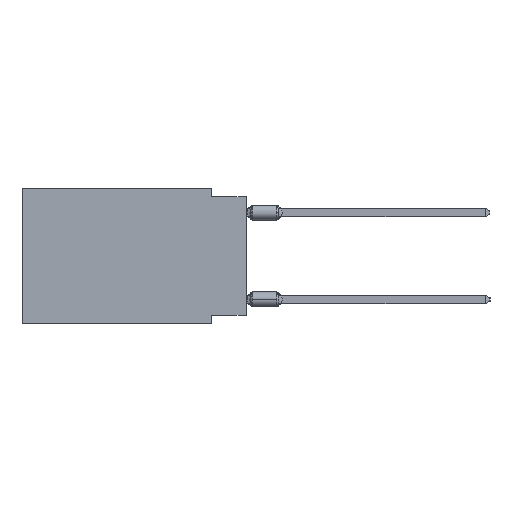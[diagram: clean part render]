
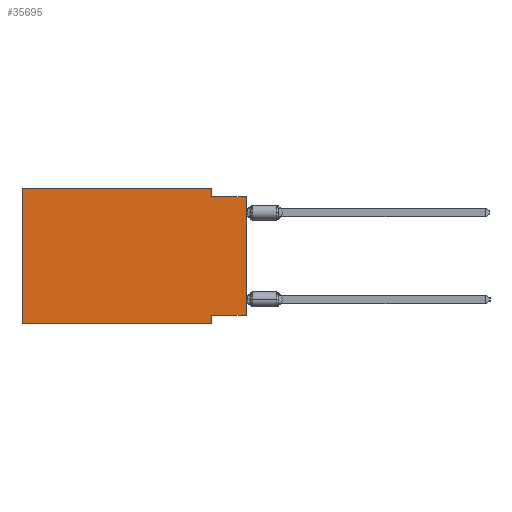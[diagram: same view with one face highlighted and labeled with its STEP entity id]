
A CAD part, left-side view. The second image highlights one B-rep face of the part: STEP entity #35695.
In plain terms, the highlighted planar face has unit normal (-1, 0, 0).
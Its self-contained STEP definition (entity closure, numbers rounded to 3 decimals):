
#551 = EDGE_CURVE ( 'NONE', #41948, #16310, #34120, .T. ) ;
#929 = DIRECTION ( 'NONE',  ( 0., 0., 1. ) ) ;
#3057 = ORIENTED_EDGE ( 'NONE', *, *, #26058, .F. ) ;
#3910 = CARTESIAN_POINT ( 'NONE',  ( 0., 2.54, -9.906 ) ) ;
#4034 = LINE ( 'NONE', #36126, #18903 ) ;
#4175 = VECTOR ( 'NONE', #14266, 1000. ) ;
#4250 = VERTEX_POINT ( 'NONE', #23758 ) ;
#4418 = DIRECTION ( 'NONE',  ( 0., -1., 0. ) ) ;
#5272 = ORIENTED_EDGE ( 'NONE', *, *, #21937, .F. ) ;
#5282 = CARTESIAN_POINT ( 'NONE',  ( 0., 2.54, 0. ) ) ;
#10532 = VECTOR ( 'NONE', #23453, 1000. ) ;
#10902 = PLANE ( 'NONE',  #42151 ) ;
#11302 = VECTOR ( 'NONE', #32524, 1000. ) ;
#14081 = VERTEX_POINT ( 'NONE', #3910 ) ;
#14266 = DIRECTION ( 'NONE',  ( 0., 1., 0. ) ) ;
#15259 = FACE_OUTER_BOUND ( 'NONE', #35864, .T. ) ;
#15515 = LINE ( 'NONE', #34306, #42172 ) ;
#15875 = VERTEX_POINT ( 'NONE', #19026 ) ;
#16050 = CARTESIAN_POINT ( 'NONE',  ( 0., 16.383, 0. ) ) ;
#16310 = VERTEX_POINT ( 'NONE', #20980 ) ;
#16678 = CARTESIAN_POINT ( 'NONE',  ( 0., 2.54, 0. ) ) ;
#16732 = LINE ( 'NONE', #36008, #33087 ) ;
#17043 = VECTOR ( 'NONE', #48157, 1000. ) ;
#18903 = VECTOR ( 'NONE', #929, 1000. ) ;
#19026 = CARTESIAN_POINT ( 'NONE',  ( 0., 0., -9.271 ) ) ;
#20980 = CARTESIAN_POINT ( 'NONE',  ( 0., 0., -0.635 ) ) ;
#21937 = EDGE_CURVE ( 'NONE', #40856, #30535, #4034, .T. ) ;
#22571 = CARTESIAN_POINT ( 'NONE',  ( 0., 0., -0.635 ) ) ;
#22885 = VECTOR ( 'NONE', #46199, 1000. ) ;
#23201 = LINE ( 'NONE', #26546, #10532 ) ;
#23453 = DIRECTION ( 'NONE',  ( 0., 0., 1. ) ) ;
#23758 = CARTESIAN_POINT ( 'NONE',  ( 0., 2.54, -9.271 ) ) ;
#24094 = CARTESIAN_POINT ( 'NONE',  ( 0., 16.383, 0. ) ) ;
#25014 = LINE ( 'NONE', #16050, #17043 ) ;
#26013 = ORIENTED_EDGE ( 'NONE', *, *, #44703, .F. ) ;
#26058 = EDGE_CURVE ( 'NONE', #4250, #14081, #15515, .T. ) ;
#26546 = CARTESIAN_POINT ( 'NONE',  ( 0., 0., 0. ) ) ;
#26577 = CARTESIAN_POINT ( 'NONE',  ( 0., 16.383, 0. ) ) ;
#28498 = ORIENTED_EDGE ( 'NONE', *, *, #551, .F. ) ;
#30317 = VERTEX_POINT ( 'NONE', #16678 ) ;
#30535 = VERTEX_POINT ( 'NONE', #24094 ) ;
#30918 = DIRECTION ( 'NONE',  ( 0., 0., -1. ) ) ;
#32524 = DIRECTION ( 'NONE',  ( 0., 0., -1. ) ) ;
#33087 = VECTOR ( 'NONE', #4418, 1000. ) ;
#34120 = LINE ( 'NONE', #22571, #22885 ) ;
#34306 = CARTESIAN_POINT ( 'NONE',  ( 0., 2.54, -9.906 ) ) ;
#34612 = ORIENTED_EDGE ( 'NONE', *, *, #45403, .T. ) ;
#34813 = DIRECTION ( 'NONE',  ( 0., 0., -1. ) ) ;
#35695 = ADVANCED_FACE ( 'NONE', ( #15259 ), #10902, .F. ) ;
#35864 = EDGE_LOOP ( 'NONE', ( #34612, #28498, #26013, #45335, #5272, #40911, #3057, #37621 ) ) ;
#36008 = CARTESIAN_POINT ( 'NONE',  ( 0., 16.383, -9.906 ) ) ;
#36126 = CARTESIAN_POINT ( 'NONE',  ( 0., 16.383, 0. ) ) ;
#37117 = EDGE_CURVE ( 'NONE', #40856, #14081, #16732, .T. ) ;
#37621 = ORIENTED_EDGE ( 'NONE', *, *, #50112, .F. ) ;
#37654 = LINE ( 'NONE', #45623, #4175 ) ;
#38395 = CARTESIAN_POINT ( 'NONE',  ( 0., 2.54, -0.635 ) ) ;
#40260 = LINE ( 'NONE', #5282, #11302 ) ;
#40856 = VERTEX_POINT ( 'NONE', #43505 ) ;
#40911 = ORIENTED_EDGE ( 'NONE', *, *, #37117, .T. ) ;
#41948 = VERTEX_POINT ( 'NONE', #38395 ) ;
#42151 = AXIS2_PLACEMENT_3D ( 'NONE', #26577, #42768, #30918 ) ;
#42172 = VECTOR ( 'NONE', #34813, 1000. ) ;
#42768 = DIRECTION ( 'NONE',  ( 1., 0., 0. ) ) ;
#43505 = CARTESIAN_POINT ( 'NONE',  ( 0., 16.383, -9.906 ) ) ;
#44703 = EDGE_CURVE ( 'NONE', #30317, #41948, #40260, .T. ) ;
#45055 = EDGE_CURVE ( 'NONE', #30535, #30317, #25014, .T. ) ;
#45335 = ORIENTED_EDGE ( 'NONE', *, *, #45055, .F. ) ;
#45403 = EDGE_CURVE ( 'NONE', #15875, #16310, #23201, .T. ) ;
#45623 = CARTESIAN_POINT ( 'NONE',  ( 0., 0., -9.271 ) ) ;
#46199 = DIRECTION ( 'NONE',  ( 0., -1., 0. ) ) ;
#48157 = DIRECTION ( 'NONE',  ( 0., -1., 0. ) ) ;
#50112 = EDGE_CURVE ( 'NONE', #15875, #4250, #37654, .T. ) ;
